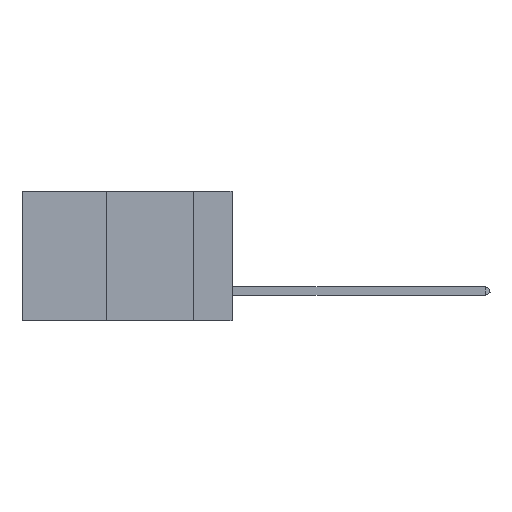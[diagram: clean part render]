
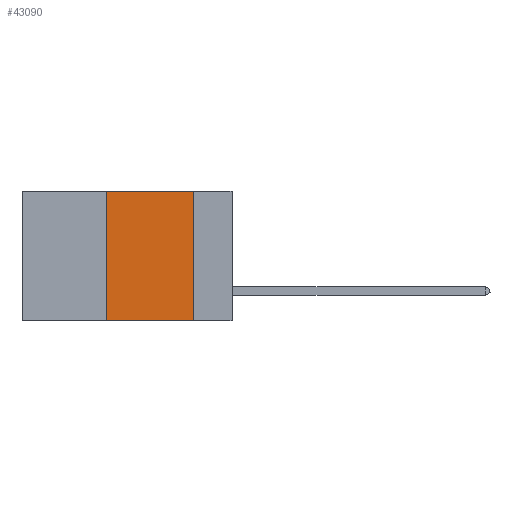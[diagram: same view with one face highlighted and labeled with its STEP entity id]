
A CAD part, left-side view. The second image highlights one B-rep face of the part: STEP entity #43090.
In plain terms, the highlighted planar face has unit normal (-1, 0, 0).
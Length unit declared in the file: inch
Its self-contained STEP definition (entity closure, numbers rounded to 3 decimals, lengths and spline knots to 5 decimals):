
#1160 = CARTESIAN_POINT ( 'NONE',  ( 0., 0.36, 0. ) ) ;
#2429 = PLANE ( 'NONE',  #5996 ) ;
#2639 = DIRECTION ( 'NONE',  ( 0., -1., 0. ) ) ;
#5292 = ORIENTED_EDGE ( 'NONE', *, *, #32869, .F. ) ;
#5821 = EDGE_LOOP ( 'NONE', ( #28429, #8490, #5292, #24096 ) ) ;
#5838 = DIRECTION ( 'NONE',  ( 1., 0., 0. ) ) ;
#5996 = AXIS2_PLACEMENT_3D ( 'NONE', #25973, #5838, #29370 ) ;
#6962 = CARTESIAN_POINT ( 'NONE',  ( 0., 0.11, 0. ) ) ;
#7286 = DIRECTION ( 'NONE',  ( 0., -1., 0. ) ) ;
#8490 = ORIENTED_EDGE ( 'NONE', *, *, #26784, .F. ) ;
#8776 = FACE_OUTER_BOUND ( 'NONE', #5821, .T. ) ;
#9314 = LINE ( 'NONE', #40034, #11914 ) ;
#10130 = DIRECTION ( 'NONE',  ( 0., 0., 1. ) ) ;
#10833 = CARTESIAN_POINT ( 'NONE',  ( 0., 0.11, 0. ) ) ;
#11914 = VECTOR ( 'NONE', #10130, 39.37008 ) ;
#13306 = CARTESIAN_POINT ( 'NONE',  ( 0., 0.6, 0. ) ) ;
#13796 = LINE ( 'NONE', #13306, #43129 ) ;
#14970 = VECTOR ( 'NONE', #18018, 39.37008 ) ;
#18018 = DIRECTION ( 'NONE',  ( 0., 0., -1. ) ) ;
#19380 = VERTEX_POINT ( 'NONE', #24688 ) ;
#20647 = CARTESIAN_POINT ( 'NONE',  ( 0., 0.6, -0.37 ) ) ;
#21659 = VERTEX_POINT ( 'NONE', #30940 ) ;
#22484 = VECTOR ( 'NONE', #7286, 39.37008 ) ;
#24096 = ORIENTED_EDGE ( 'NONE', *, *, #31459, .T. ) ;
#24398 = VERTEX_POINT ( 'NONE', #1160 ) ;
#24688 = CARTESIAN_POINT ( 'NONE',  ( 0., 0.36, -0.37 ) ) ;
#25973 = CARTESIAN_POINT ( 'NONE',  ( 0., 0.6, 0. ) ) ;
#26784 = EDGE_CURVE ( 'NONE', #24398, #31230, #13796, .T. ) ;
#28429 = ORIENTED_EDGE ( 'NONE', *, *, #38910, .F. ) ;
#29370 = DIRECTION ( 'NONE',  ( 0., 0., -1. ) ) ;
#30940 = CARTESIAN_POINT ( 'NONE',  ( 0., 0.11, -0.37 ) ) ;
#31230 = VERTEX_POINT ( 'NONE', #6962 ) ;
#31459 = EDGE_CURVE ( 'NONE', #19380, #21659, #32453, .T. ) ;
#31787 = LINE ( 'NONE', #10833, #14970 ) ;
#32453 = LINE ( 'NONE', #20647, #22484 ) ;
#32869 = EDGE_CURVE ( 'NONE', #19380, #24398, #9314, .T. ) ;
#38910 = EDGE_CURVE ( 'NONE', #31230, #21659, #31787, .T. ) ;
#40034 = CARTESIAN_POINT ( 'NONE',  ( 0., 0.36, 0. ) ) ;
#43090 = ADVANCED_FACE ( 'NONE', ( #8776 ), #2429, .F. ) ;
#43129 = VECTOR ( 'NONE', #2639, 39.37008 ) ;
